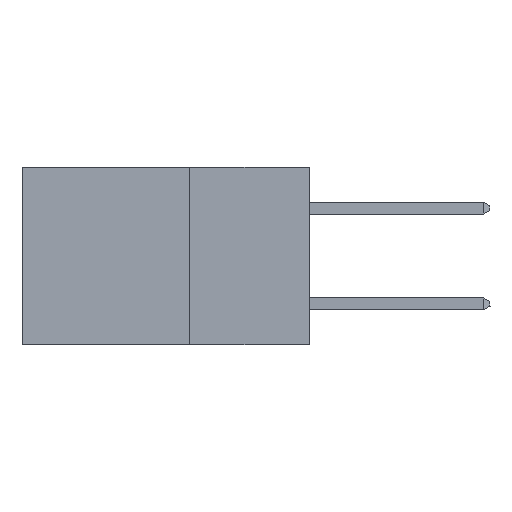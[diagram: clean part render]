
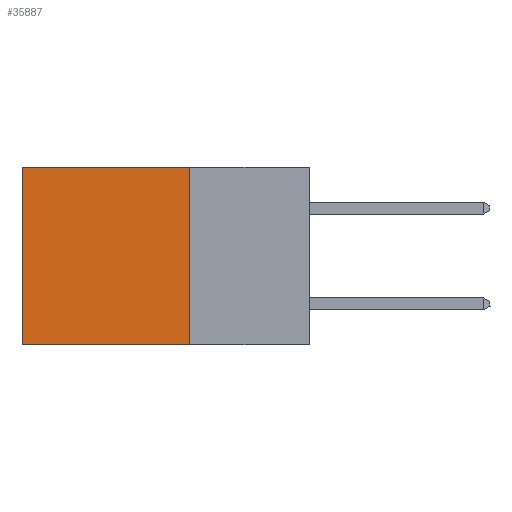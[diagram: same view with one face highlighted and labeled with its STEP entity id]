
A CAD part, left-side view. The second image highlights one B-rep face of the part: STEP entity #35887.
In plain terms, the highlighted planar face has unit normal (-1, 0, 0).
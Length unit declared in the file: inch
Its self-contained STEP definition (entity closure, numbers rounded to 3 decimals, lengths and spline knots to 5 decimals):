
#3516 = DIRECTION ( 'NONE',  ( 0., 0., -1. ) ) ;
#3882 = CARTESIAN_POINT ( 'NONE',  ( 0.2875, 0.25, 0. ) ) ;
#4071 = ORIENTED_EDGE ( 'NONE', *, *, #12632, .F. ) ;
#5203 = EDGE_CURVE ( 'NONE', #14618, #5574, #12673, .T. ) ;
#5417 = DIRECTION ( 'NONE',  ( 0., 0., -1. ) ) ;
#5574 = VERTEX_POINT ( 'NONE', #32788 ) ;
#5833 = EDGE_LOOP ( 'NONE', ( #25202, #17644, #4071, #9034 ) ) ;
#7049 = VECTOR ( 'NONE', #5417, 39.37008 ) ;
#9034 = ORIENTED_EDGE ( 'NONE', *, *, #11051, .T. ) ;
#9496 = DIRECTION ( 'NONE',  ( 0., 1., 0. ) ) ;
#9607 = VECTOR ( 'NONE', #20612, 39.37008 ) ;
#10636 = CARTESIAN_POINT ( 'NONE',  ( 0.2875, 0.25, 0. ) ) ;
#11051 = EDGE_CURVE ( 'NONE', #27708, #14618, #17484, .T. ) ;
#12459 = CARTESIAN_POINT ( 'NONE',  ( 0.2875, 0.25, 0. ) ) ;
#12632 = EDGE_CURVE ( 'NONE', #27708, #15297, #33264, .T. ) ;
#12673 = LINE ( 'NONE', #13763, #13233 ) ;
#13233 = VECTOR ( 'NONE', #30654, 39.37008 ) ;
#13763 = CARTESIAN_POINT ( 'NONE',  ( 0.2875, 0.6, 0. ) ) ;
#14618 = VERTEX_POINT ( 'NONE', #36230 ) ;
#14769 = VECTOR ( 'NONE', #9496, 39.37008 ) ;
#15297 = VERTEX_POINT ( 'NONE', #23720 ) ;
#17484 = LINE ( 'NONE', #12459, #14769 ) ;
#17644 = ORIENTED_EDGE ( 'NONE', *, *, #30237, .F. ) ;
#20612 = DIRECTION ( 'NONE',  ( 0., 1., 0. ) ) ;
#20965 = DIRECTION ( 'NONE',  ( 1., 0., 0. ) ) ;
#23317 = CARTESIAN_POINT ( 'NONE',  ( 0.2875, 0.25, 0. ) ) ;
#23720 = CARTESIAN_POINT ( 'NONE',  ( 0.2875, 0.25, -0.37 ) ) ;
#25202 = ORIENTED_EDGE ( 'NONE', *, *, #5203, .T. ) ;
#27708 = VERTEX_POINT ( 'NONE', #23317 ) ;
#28782 = FACE_OUTER_BOUND ( 'NONE', #5833, .T. ) ;
#29130 = LINE ( 'NONE', #34706, #9607 ) ;
#29131 = PLANE ( 'NONE',  #33607 ) ;
#30237 = EDGE_CURVE ( 'NONE', #15297, #5574, #29130, .T. ) ;
#30654 = DIRECTION ( 'NONE',  ( 0., 0., -1. ) ) ;
#32788 = CARTESIAN_POINT ( 'NONE',  ( 0.2875, 0.6, -0.37 ) ) ;
#33264 = LINE ( 'NONE', #10636, #7049 ) ;
#33607 = AXIS2_PLACEMENT_3D ( 'NONE', #3882, #20965, #3516 ) ;
#34706 = CARTESIAN_POINT ( 'NONE',  ( 0.2875, 0.25, -0.37 ) ) ;
#35887 = ADVANCED_FACE ( 'NONE', ( #28782 ), #29131, .F. ) ;
#36230 = CARTESIAN_POINT ( 'NONE',  ( 0.2875, 0.6, 0. ) ) ;
